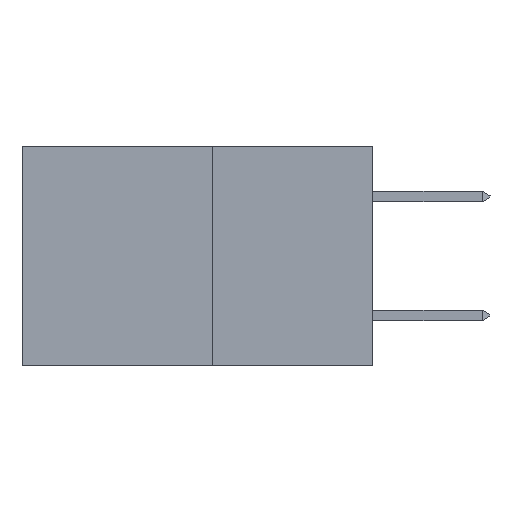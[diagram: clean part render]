
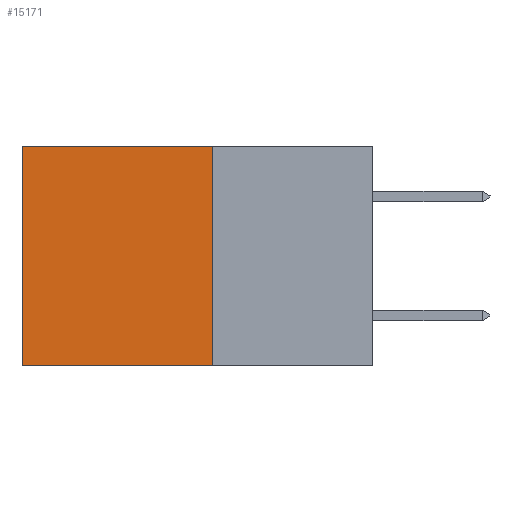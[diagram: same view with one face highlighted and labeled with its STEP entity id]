
A CAD part, left-side view. The second image highlights one B-rep face of the part: STEP entity #15171.
In plain terms, the highlighted planar face has unit normal (-1, 0, 0).
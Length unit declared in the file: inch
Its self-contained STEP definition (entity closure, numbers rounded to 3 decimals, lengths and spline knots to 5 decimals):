
#117 = DIRECTION ( 'NONE',  ( 0., 0., -1. ) ) ;
#721 = VERTEX_POINT ( 'NONE', #14272 ) ;
#1407 = CARTESIAN_POINT ( 'NONE',  ( 0.277, 0.27, -0.37 ) ) ;
#1761 = VECTOR ( 'NONE', #12821, 39.37008 ) ;
#1766 = AXIS2_PLACEMENT_3D ( 'NONE', #4510, #10960, #3285 ) ;
#1996 = PLANE ( 'NONE',  #1766 ) ;
#2342 = EDGE_CURVE ( 'NONE', #15654, #5842, #14945, .T. ) ;
#3285 = DIRECTION ( 'NONE',  ( 0., 0., -1. ) ) ;
#3353 = DIRECTION ( 'NONE',  ( 0., 1., 0. ) ) ;
#3521 = ORIENTED_EDGE ( 'NONE', *, *, #8342, .F. ) ;
#3785 = CARTESIAN_POINT ( 'NONE',  ( 0.277, 0.27, 0. ) ) ;
#3914 = ORIENTED_EDGE ( 'NONE', *, *, #2342, .T. ) ;
#4264 = CARTESIAN_POINT ( 'NONE',  ( 0.277, 0.27, -0.37 ) ) ;
#4510 = CARTESIAN_POINT ( 'NONE',  ( 0.277, 0.27, -0.37 ) ) ;
#5065 = CARTESIAN_POINT ( 'NONE',  ( 0.277, 0.59, 0. ) ) ;
#5842 = VERTEX_POINT ( 'NONE', #5065 ) ;
#6341 = VECTOR ( 'NONE', #3353, 39.37008 ) ;
#6757 = LINE ( 'NONE', #11029, #6341 ) ;
#7273 = FACE_OUTER_BOUND ( 'NONE', #11979, .T. ) ;
#7764 = VERTEX_POINT ( 'NONE', #4264 ) ;
#8342 = EDGE_CURVE ( 'NONE', #15654, #7764, #15489, .T. ) ;
#8464 = VECTOR ( 'NONE', #13504, 39.37008 ) ;
#8559 = LINE ( 'NONE', #15290, #11495 ) ;
#10047 = EDGE_CURVE ( 'NONE', #7764, #721, #6757, .T. ) ;
#10627 = EDGE_CURVE ( 'NONE', #5842, #721, #8559, .T. ) ;
#10960 = DIRECTION ( 'NONE',  ( 1., 0., 0. ) ) ;
#11029 = CARTESIAN_POINT ( 'NONE',  ( 0.277, 0.27, -0.37 ) ) ;
#11495 = VECTOR ( 'NONE', #117, 39.37008 ) ;
#11979 = EDGE_LOOP ( 'NONE', ( #12076, #13215, #3521, #3914 ) ) ;
#12076 = ORIENTED_EDGE ( 'NONE', *, *, #10627, .T. ) ;
#12821 = DIRECTION ( 'NONE',  ( 0., 0., -1. ) ) ;
#13060 = CARTESIAN_POINT ( 'NONE',  ( 0.277, 0.27, 0. ) ) ;
#13215 = ORIENTED_EDGE ( 'NONE', *, *, #10047, .F. ) ;
#13504 = DIRECTION ( 'NONE',  ( 0., 1., 0. ) ) ;
#14272 = CARTESIAN_POINT ( 'NONE',  ( 0.277, 0.59, -0.37 ) ) ;
#14945 = LINE ( 'NONE', #3785, #8464 ) ;
#15171 = ADVANCED_FACE ( 'NONE', ( #7273 ), #1996, .F. ) ;
#15290 = CARTESIAN_POINT ( 'NONE',  ( 0.277, 0.59, -0.37 ) ) ;
#15489 = LINE ( 'NONE', #1407, #1761 ) ;
#15654 = VERTEX_POINT ( 'NONE', #13060 ) ;
